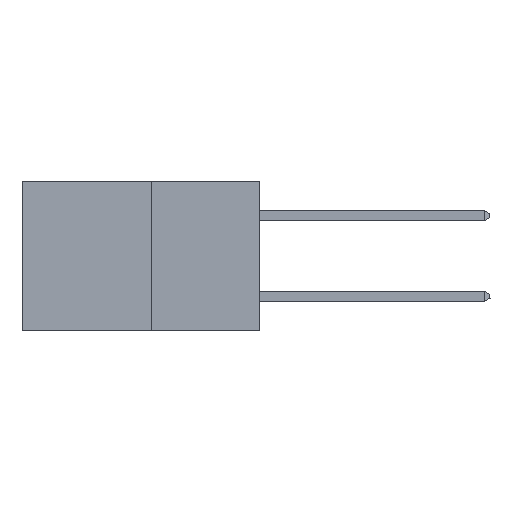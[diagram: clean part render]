
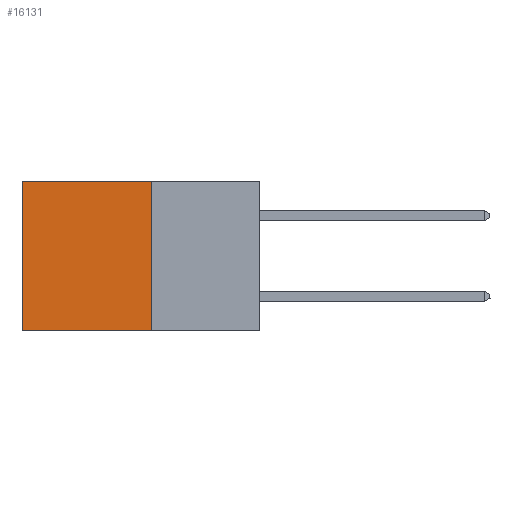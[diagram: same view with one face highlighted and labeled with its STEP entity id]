
A CAD part, left-side view. The second image highlights one B-rep face of the part: STEP entity #16131.
In plain terms, the highlighted planar face has unit normal (-1, 0, 0).
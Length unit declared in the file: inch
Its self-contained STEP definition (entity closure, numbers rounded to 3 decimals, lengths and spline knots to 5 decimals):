
#559 = CARTESIAN_POINT ( 'NONE',  ( 0.277, 0.27, 0. ) ) ;
#1785 = EDGE_CURVE ( 'NONE', #19962, #9052, #7266, .T. ) ;
#1861 = VECTOR ( 'NONE', #21713, 39.37008 ) ;
#2311 = EDGE_LOOP ( 'NONE', ( #7010, #26280, #6777, #22404 ) ) ;
#3395 = DIRECTION ( 'NONE',  ( 0., 0., -1. ) ) ;
#3401 = VECTOR ( 'NONE', #17256, 39.37008 ) ;
#3705 = CARTESIAN_POINT ( 'NONE',  ( 0.277, 0.27, -0.37 ) ) ;
#4345 = VERTEX_POINT ( 'NONE', #559 ) ;
#5730 = PLANE ( 'NONE',  #24516 ) ;
#5996 = CARTESIAN_POINT ( 'NONE',  ( 0.277, 0.27, -0.37 ) ) ;
#6777 = ORIENTED_EDGE ( 'NONE', *, *, #7079, .F. ) ;
#6823 = VERTEX_POINT ( 'NONE', #5996 ) ;
#7010 = ORIENTED_EDGE ( 'NONE', *, *, #1785, .T. ) ;
#7079 = EDGE_CURVE ( 'NONE', #4345, #6823, #14141, .T. ) ;
#7266 = LINE ( 'NONE', #24169, #1861 ) ;
#7758 = DIRECTION ( 'NONE',  ( 1., 0., 0. ) ) ;
#8798 = EDGE_CURVE ( 'NONE', #4345, #19962, #10227, .T. ) ;
#9052 = VERTEX_POINT ( 'NONE', #12903 ) ;
#9281 = CARTESIAN_POINT ( 'NONE',  ( 0.277, 0.59, 0. ) ) ;
#10227 = LINE ( 'NONE', #20435, #19845 ) ;
#11108 = EDGE_CURVE ( 'NONE', #6823, #9052, #13641, .T. ) ;
#12903 = CARTESIAN_POINT ( 'NONE',  ( 0.277, 0.59, -0.37 ) ) ;
#13641 = LINE ( 'NONE', #25545, #3401 ) ;
#14141 = LINE ( 'NONE', #3705, #18311 ) ;
#16131 = ADVANCED_FACE ( 'NONE', ( #16406 ), #5730, .F. ) ;
#16406 = FACE_OUTER_BOUND ( 'NONE', #2311, .T. ) ;
#17256 = DIRECTION ( 'NONE',  ( 0., 1., 0. ) ) ;
#18311 = VECTOR ( 'NONE', #3395, 39.37008 ) ;
#18386 = DIRECTION ( 'NONE',  ( 0., 1., 0. ) ) ;
#19845 = VECTOR ( 'NONE', #18386, 39.37008 ) ;
#19962 = VERTEX_POINT ( 'NONE', #9281 ) ;
#20060 = CARTESIAN_POINT ( 'NONE',  ( 0.277, 0.27, -0.37 ) ) ;
#20435 = CARTESIAN_POINT ( 'NONE',  ( 0.277, 0.27, 0. ) ) ;
#21713 = DIRECTION ( 'NONE',  ( 0., 0., -1. ) ) ;
#22137 = DIRECTION ( 'NONE',  ( 0., 0., -1. ) ) ;
#22404 = ORIENTED_EDGE ( 'NONE', *, *, #8798, .T. ) ;
#24169 = CARTESIAN_POINT ( 'NONE',  ( 0.277, 0.59, -0.37 ) ) ;
#24516 = AXIS2_PLACEMENT_3D ( 'NONE', #20060, #7758, #22137 ) ;
#25545 = CARTESIAN_POINT ( 'NONE',  ( 0.277, 0.27, -0.37 ) ) ;
#26280 = ORIENTED_EDGE ( 'NONE', *, *, #11108, .F. ) ;
